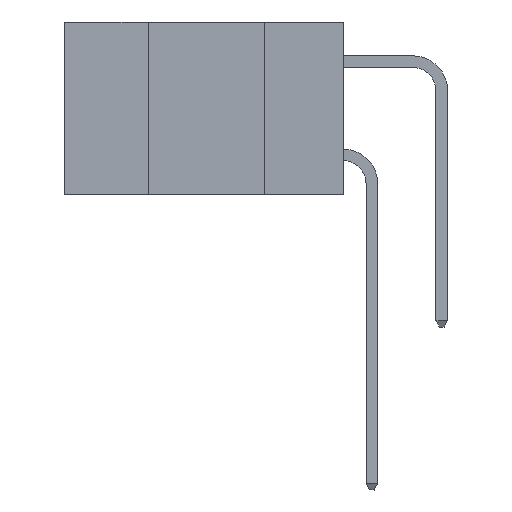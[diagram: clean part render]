
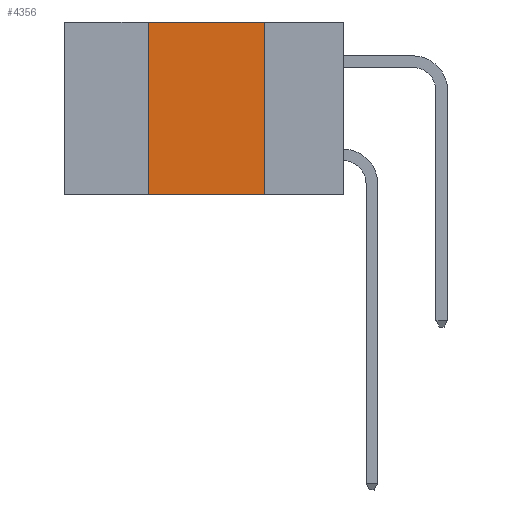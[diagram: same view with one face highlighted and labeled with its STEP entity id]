
A CAD part, left-side view. The second image highlights one B-rep face of the part: STEP entity #4356.
In plain terms, the highlighted planar face has unit normal (-1, 0, 0).
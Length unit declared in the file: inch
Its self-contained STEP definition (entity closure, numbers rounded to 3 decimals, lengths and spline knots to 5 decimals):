
#183 = CARTESIAN_POINT ( 'NONE',  ( 0., 0.6, 0. ) ) ;
#555 = CARTESIAN_POINT ( 'NONE',  ( 0., 0.6, -0.37 ) ) ;
#1083 = CARTESIAN_POINT ( 'NONE',  ( 0., 0.17, 0. ) ) ;
#1162 = VECTOR ( 'NONE', #2626, 39.37008 ) ;
#1243 = DIRECTION ( 'NONE',  ( 1., 0., 0. ) ) ;
#1419 = AXIS2_PLACEMENT_3D ( 'NONE', #183, #1243, #8372 ) ;
#1593 = ORIENTED_EDGE ( 'NONE', *, *, #8455, .F. ) ;
#2116 = CARTESIAN_POINT ( 'NONE',  ( 0., 0.17, -0.37 ) ) ;
#2247 = EDGE_CURVE ( 'NONE', #4923, #2784, #7761, .T. ) ;
#2488 = CARTESIAN_POINT ( 'NONE',  ( 0., 0.42, -0.37 ) ) ;
#2626 = DIRECTION ( 'NONE',  ( 0., -1., 0. ) ) ;
#2784 = VERTEX_POINT ( 'NONE', #3543 ) ;
#2935 = DIRECTION ( 'NONE',  ( 0., 0., 1. ) ) ;
#3050 = DIRECTION ( 'NONE',  ( 0., 0., -1. ) ) ;
#3080 = DIRECTION ( 'NONE',  ( 0., -1., 0. ) ) ;
#3543 = CARTESIAN_POINT ( 'NONE',  ( 0., 0.17, -0.37 ) ) ;
#4356 = ADVANCED_FACE ( 'NONE', ( #12595 ), #6304, .F. ) ;
#4923 = VERTEX_POINT ( 'NONE', #2488 ) ;
#5404 = VECTOR ( 'NONE', #2935, 39.37008 ) ;
#6304 = PLANE ( 'NONE',  #1419 ) ;
#6389 = EDGE_CURVE ( 'NONE', #11333, #9525, #8153, .T. ) ;
#6812 = EDGE_CURVE ( 'NONE', #4923, #11333, #13031, .T. ) ;
#7084 = CARTESIAN_POINT ( 'NONE',  ( 0., 0.42, -0.37 ) ) ;
#7761 = LINE ( 'NONE', #555, #1162 ) ;
#8153 = LINE ( 'NONE', #12233, #12388 ) ;
#8372 = DIRECTION ( 'NONE',  ( 0., 0., -1. ) ) ;
#8455 = EDGE_CURVE ( 'NONE', #9525, #2784, #11270, .T. ) ;
#8532 = CARTESIAN_POINT ( 'NONE',  ( 0., 0.42, 0. ) ) ;
#9360 = VECTOR ( 'NONE', #3050, 39.37008 ) ;
#9525 = VERTEX_POINT ( 'NONE', #1083 ) ;
#10399 = ORIENTED_EDGE ( 'NONE', *, *, #2247, .T. ) ;
#10555 = ORIENTED_EDGE ( 'NONE', *, *, #6812, .F. ) ;
#10806 = ORIENTED_EDGE ( 'NONE', *, *, #6389, .F. ) ;
#11270 = LINE ( 'NONE', #2116, #9360 ) ;
#11333 = VERTEX_POINT ( 'NONE', #8532 ) ;
#12216 = EDGE_LOOP ( 'NONE', ( #1593, #10806, #10555, #10399 ) ) ;
#12233 = CARTESIAN_POINT ( 'NONE',  ( 0., 0.6, 0. ) ) ;
#12388 = VECTOR ( 'NONE', #3080, 39.37008 ) ;
#12595 = FACE_OUTER_BOUND ( 'NONE', #12216, .T. ) ;
#13031 = LINE ( 'NONE', #7084, #5404 ) ;
